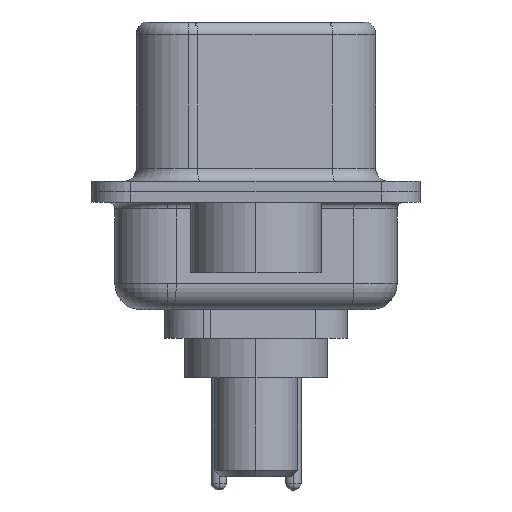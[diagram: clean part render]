
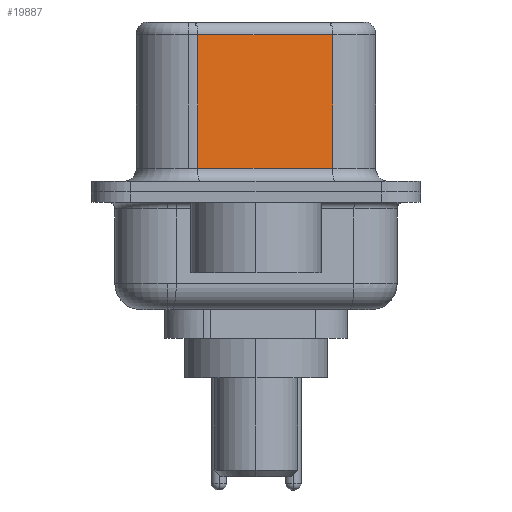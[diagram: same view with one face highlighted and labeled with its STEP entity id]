
A CAD part, left-side view. The second image highlights one B-rep face of the part: STEP entity #19887.
In plain terms, the highlighted planar face has unit normal (-0.985, -0.174, 0).
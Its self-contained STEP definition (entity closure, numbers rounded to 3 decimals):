
#971 = DIRECTION ( 'NONE',  ( -0.174, 0.985, 0. ) ) ;
#978 = EDGE_CURVE ( 'NONE', #7856, #13089, #6640, .T. ) ;
#3998 = VERTEX_POINT ( 'NONE', #5230 ) ;
#4253 = CARTESIAN_POINT ( 'NONE',  ( 4.58, -2.927, 6.02 ) ) ;
#4468 = CARTESIAN_POINT ( 'NONE',  ( 3.67, 2.233, 6.52 ) ) ;
#4534 = AXIS2_PLACEMENT_3D ( 'NONE', #20797, #11043, #971 ) ;
#5230 = CARTESIAN_POINT ( 'NONE',  ( 4.58, -2.927, 0.9 ) ) ;
#5330 = EDGE_CURVE ( 'NONE', #14103, #3998, #17919, .T. ) ;
#5400 = VECTOR ( 'NONE', #14268, 1000. ) ;
#6640 = LINE ( 'NONE', #13856, #14877 ) ;
#7729 = PLANE ( 'NONE',  #4534 ) ;
#7856 = VERTEX_POINT ( 'NONE', #4253 ) ;
#10377 = EDGE_LOOP ( 'NONE', ( #17780, #18579, #19519, #19263 ) ) ;
#11020 = LINE ( 'NONE', #4468, #15403 ) ;
#11043 = DIRECTION ( 'NONE',  ( 0.985, 0.174, 0. ) ) ;
#12296 = DIRECTION ( 'NONE',  ( 0., 0., -1. ) ) ;
#13089 = VERTEX_POINT ( 'NONE', #20706 ) ;
#13856 = CARTESIAN_POINT ( 'NONE',  ( 4.58, -2.927, 6.02 ) ) ;
#14103 = VERTEX_POINT ( 'NONE', #19206 ) ;
#14268 = DIRECTION ( 'NONE',  ( 0.174, -0.985, 0. ) ) ;
#14316 = CARTESIAN_POINT ( 'NONE',  ( 4.58, -2.927, 0.9 ) ) ;
#14877 = VECTOR ( 'NONE', #19279, 1000. ) ;
#15403 = VECTOR ( 'NONE', #15991, 1000. ) ;
#15898 = FACE_OUTER_BOUND ( 'NONE', #10377, .T. ) ;
#15991 = DIRECTION ( 'NONE',  ( 0., 0., -1. ) ) ;
#16925 = EDGE_CURVE ( 'NONE', #7856, #3998, #18918, .T. ) ;
#17780 = ORIENTED_EDGE ( 'NONE', *, *, #16925, .F. ) ;
#17919 = LINE ( 'NONE', #14316, #5400 ) ;
#18412 = VECTOR ( 'NONE', #12296, 1000. ) ;
#18579 = ORIENTED_EDGE ( 'NONE', *, *, #978, .T. ) ;
#18810 = CARTESIAN_POINT ( 'NONE',  ( 4.58, -2.927, 6.52 ) ) ;
#18918 = LINE ( 'NONE', #18810, #18412 ) ;
#19206 = CARTESIAN_POINT ( 'NONE',  ( 3.67, 2.233, 0.9 ) ) ;
#19263 = ORIENTED_EDGE ( 'NONE', *, *, #5330, .T. ) ;
#19279 = DIRECTION ( 'NONE',  ( -0.174, 0.985, 0. ) ) ;
#19519 = ORIENTED_EDGE ( 'NONE', *, *, #19888, .T. ) ;
#19887 = ADVANCED_FACE ( 'NONE', ( #15898 ), #7729, .F. ) ;
#19888 = EDGE_CURVE ( 'NONE', #13089, #14103, #11020, .T. ) ;
#20706 = CARTESIAN_POINT ( 'NONE',  ( 3.67, 2.233, 6.02 ) ) ;
#20797 = CARTESIAN_POINT ( 'NONE',  ( 4.58, -2.927, 6.52 ) ) ;
